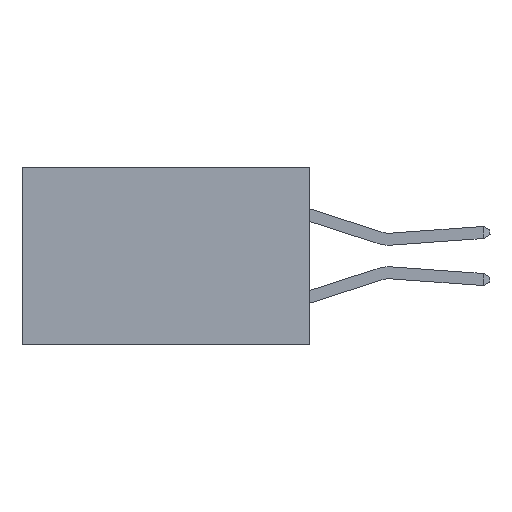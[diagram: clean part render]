
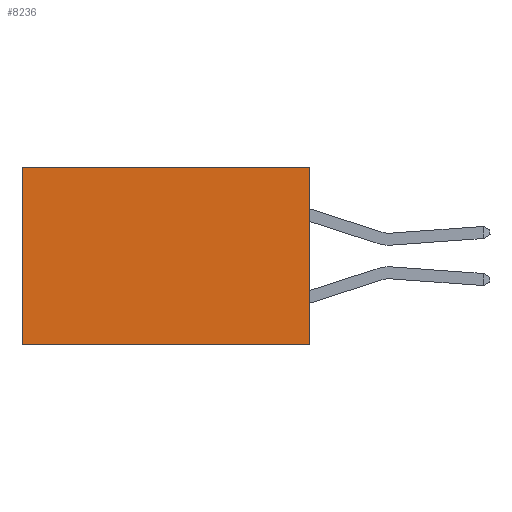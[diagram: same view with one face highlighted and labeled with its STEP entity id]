
A CAD part, left-side view. The second image highlights one B-rep face of the part: STEP entity #8236.
In plain terms, the highlighted planar face has unit normal (-1, 0, 0).
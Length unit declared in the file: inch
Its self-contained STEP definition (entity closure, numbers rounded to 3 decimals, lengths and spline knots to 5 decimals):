
#592 = LINE ( 'NONE', #10150, #3064 ) ;
#860 = DIRECTION ( 'NONE',  ( 0., 0., -1. ) ) ;
#1027 = VERTEX_POINT ( 'NONE', #2370 ) ;
#1902 = ORIENTED_EDGE ( 'NONE', *, *, #11136, .T. ) ;
#2182 = LINE ( 'NONE', #12714, #14517 ) ;
#2370 = CARTESIAN_POINT ( 'NONE',  ( 0.2615, 0., 0. ) ) ;
#2624 = FACE_OUTER_BOUND ( 'NONE', #3023, .T. ) ;
#3023 = EDGE_LOOP ( 'NONE', ( #1902, #13058, #12067, #5763 ) ) ;
#3026 = DIRECTION ( 'NONE',  ( 0., 0., -1. ) ) ;
#3064 = VECTOR ( 'NONE', #860, 39.37008 ) ;
#3719 = VECTOR ( 'NONE', #3026, 39.37008 ) ;
#4926 = LINE ( 'NONE', #11528, #13011 ) ;
#5763 = ORIENTED_EDGE ( 'NONE', *, *, #6495, .T. ) ;
#6495 = EDGE_CURVE ( 'NONE', #1027, #8756, #4926, .T. ) ;
#6537 = CARTESIAN_POINT ( 'NONE',  ( 0.2615, 0., -0.37 ) ) ;
#6888 = DIRECTION ( 'NONE',  ( 0., 0., -1. ) ) ;
#7253 = DIRECTION ( 'NONE',  ( 0., 1., 0. ) ) ;
#8236 = ADVANCED_FACE ( 'NONE', ( #2624 ), #9309, .F. ) ;
#8756 = VERTEX_POINT ( 'NONE', #13216 ) ;
#9192 = CARTESIAN_POINT ( 'NONE',  ( 0.2615, 0., -0.37 ) ) ;
#9309 = PLANE ( 'NONE',  #17511 ) ;
#10150 = CARTESIAN_POINT ( 'NONE',  ( 0.2615, 0.6, -0.37 ) ) ;
#11136 = EDGE_CURVE ( 'NONE', #8756, #12454, #592, .T. ) ;
#11528 = CARTESIAN_POINT ( 'NONE',  ( 0.2615, 0., 0. ) ) ;
#11615 = DIRECTION ( 'NONE',  ( 0., 1., 0. ) ) ;
#12067 = ORIENTED_EDGE ( 'NONE', *, *, #16377, .F. ) ;
#12454 = VERTEX_POINT ( 'NONE', #17539 ) ;
#12714 = CARTESIAN_POINT ( 'NONE',  ( 0.2615, 0., -0.37 ) ) ;
#13011 = VECTOR ( 'NONE', #11615, 39.37008 ) ;
#13058 = ORIENTED_EDGE ( 'NONE', *, *, #15536, .F. ) ;
#13216 = CARTESIAN_POINT ( 'NONE',  ( 0.2615, 0.6, 0. ) ) ;
#13321 = DIRECTION ( 'NONE',  ( 1., 0., 0. ) ) ;
#14517 = VECTOR ( 'NONE', #7253, 39.37008 ) ;
#15239 = LINE ( 'NONE', #16386, #3719 ) ;
#15536 = EDGE_CURVE ( 'NONE', #16245, #12454, #2182, .T. ) ;
#16245 = VERTEX_POINT ( 'NONE', #9192 ) ;
#16377 = EDGE_CURVE ( 'NONE', #1027, #16245, #15239, .T. ) ;
#16386 = CARTESIAN_POINT ( 'NONE',  ( 0.2615, 0., -0.37 ) ) ;
#17511 = AXIS2_PLACEMENT_3D ( 'NONE', #6537, #13321, #6888 ) ;
#17539 = CARTESIAN_POINT ( 'NONE',  ( 0.2615, 0.6, -0.37 ) ) ;
